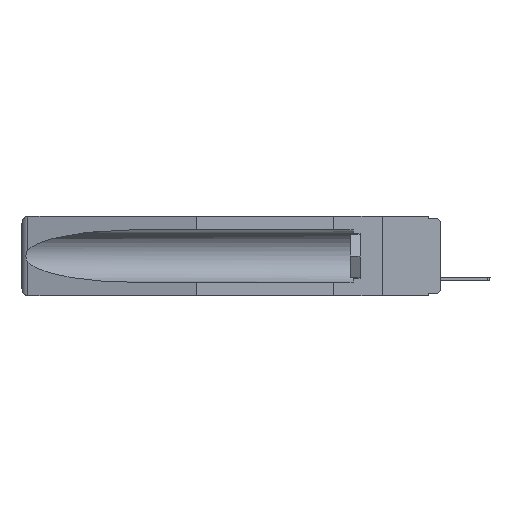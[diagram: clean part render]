
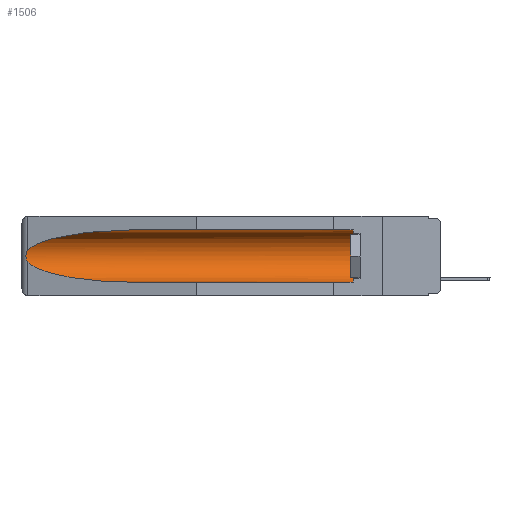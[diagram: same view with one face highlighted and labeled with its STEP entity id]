
A CAD part, left-side view. The second image highlights one B-rep face of the part: STEP entity #1506.
In plain terms, the highlighted cylindrical face has radius 2.857 mm (diameter 5.715 mm), a partial arc.
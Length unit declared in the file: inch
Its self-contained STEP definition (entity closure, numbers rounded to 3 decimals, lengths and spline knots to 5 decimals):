
#225 = EDGE_LOOP ( 'NONE', ( #8158, #10913, #3155, #18126, #15977, #18020 ) ) ;
#439 = CARTESIAN_POINT ( 'NONE',  ( 0.155, -0.30754, -0.1715 ) ) ;
#495 = VECTOR ( 'NONE', #9731, 39.37008 ) ;
#698 = VERTEX_POINT ( 'NONE', #2184 ) ;
#1495 = B_SPLINE_CURVE_WITH_KNOTS ( 'NONE', 3,
 ( #19013, #11004, #4889, #17435, #8050, #17637, #9513, #11315, #9321, #3001 ),
 .UNSPECIFIED., .F., .F.,
 ( 4, 2, 2, 2, 4 ),
 ( 0., 0.00029, 0.00058, 0.00087, 0.00117 ),
 .UNSPECIFIED. ) ;
#1506 = ADVANCED_FACE ( 'NONE', ( #10110 ), #15174, .F. ) ;
#1785 = VERTEX_POINT ( 'NONE', #9872 ) ;
#1948 =( BOUNDED_CURVE ( )  B_SPLINE_CURVE ( 3, ( #9171, #2658, #17506, #13929 ),
 .UNSPECIFIED., .F., .T. ) 
 B_SPLINE_CURVE_WITH_KNOTS ( ( 4, 4 ),
 ( 4.71239, 6.08839 ),
 .UNSPECIFIED. ) 
 CURVE ( )  GEOMETRIC_REPRESENTATION_ITEM ( )  RATIONAL_B_SPLINE_CURVE ( ( 1., 0.848, 0.848, 1. ) ) 
 REPRESENTATION_ITEM ( '' )  );
#2184 = CARTESIAN_POINT ( 'NONE',  ( 0.26537, 1.52718, -0.19328 ) ) ;
#2658 = CARTESIAN_POINT ( 'NONE',  ( 0.21114, 1.30732, -0.059 ) ) ;
#3001 = CARTESIAN_POINT ( 'NONE',  ( 0.26537, 1.52718, -0.19328 ) ) ;
#3155 = ORIENTED_EDGE ( 'NONE', *, *, #18016, .T. ) ;
#3371 = EDGE_CURVE ( 'NONE', #20706, #1785, #8905, .T. ) ;
#3880 = CARTESIAN_POINT ( 'NONE',  ( 0.25451, 1.48313, -0.24835 ) ) ;
#4019 = DIRECTION ( 'NONE',  ( 0., 1., 0. ) ) ;
#4889 = CARTESIAN_POINT ( 'NONE',  ( 0.26654, 1.53092, -0.15636 ) ) ;
#5355 = EDGE_CURVE ( 'NONE', #11355, #698, #1495, .T. ) ;
#6370 = CARTESIAN_POINT ( 'NONE',  ( 0.155, 1.07973, -0.284 ) ) ;
#6860 = DIRECTION ( 'NONE',  ( 0., 0., 1. ) ) ;
#7137 = CARTESIAN_POINT ( 'NONE',  ( 0.21114, 1.30732, -0.284 ) ) ;
#7166 = AXIS2_PLACEMENT_3D ( 'NONE', #439, #4019, #6860 ) ;
#7310 = EDGE_CURVE ( 'NONE', #20706, #19243, #8266, .T. ) ;
#7589 = EDGE_CURVE ( 'NONE', #16538, #11355, #1948, .T. ) ;
#7983 = CARTESIAN_POINT ( 'NONE',  ( 0.155, 1.07973, -0.059 ) ) ;
#8035 = LINE ( 'NONE', #16051, #13643 ) ;
#8050 = CARTESIAN_POINT ( 'NONE',  ( 0.2675, 1.53308, -0.16763 ) ) ;
#8158 = ORIENTED_EDGE ( 'NONE', *, *, #7589, .T. ) ;
#8266 = LINE ( 'NONE', #17845, #495 ) ;
#8820 = CARTESIAN_POINT ( 'NONE',  ( 0.26537, 1.52718, -0.19328 ) ) ;
#8905 = CIRCLE ( 'NONE', #10238, 0.1125 ) ;
#9171 = CARTESIAN_POINT ( 'NONE',  ( 0.155, 1.07973, -0.059 ) ) ;
#9321 = CARTESIAN_POINT ( 'NONE',  ( 0.26597, 1.5296, -0.19026 ) ) ;
#9513 = CARTESIAN_POINT ( 'NONE',  ( 0.2673, 1.53269, -0.17917 ) ) ;
#9731 = DIRECTION ( 'NONE',  ( 0., 1., 0. ) ) ;
#9872 = CARTESIAN_POINT ( 'NONE',  ( 0.155, 0.126, -0.059 ) ) ;
#10110 = FACE_OUTER_BOUND ( 'NONE', #225, .T. ) ;
#10238 = AXIS2_PLACEMENT_3D ( 'NONE', #18301, #14626, #19668 ) ;
#10538 =( BOUNDED_CURVE ( )  B_SPLINE_CURVE ( 3, ( #8820, #3880, #7137, #15049 ),
 .UNSPECIFIED., .F., .T. ) 
 B_SPLINE_CURVE_WITH_KNOTS ( ( 4, 4 ),
 ( 0.1948, 1.5708 ),
 .UNSPECIFIED. ) 
 CURVE ( )  GEOMETRIC_REPRESENTATION_ITEM ( )  RATIONAL_B_SPLINE_CURVE ( ( 1., 0.848, 0.848, 1. ) ) 
 REPRESENTATION_ITEM ( '' )  );
#10913 = ORIENTED_EDGE ( 'NONE', *, *, #5355, .T. ) ;
#11004 = CARTESIAN_POINT ( 'NONE',  ( 0.26597, 1.52961, -0.15275 ) ) ;
#11315 = CARTESIAN_POINT ( 'NONE',  ( 0.26655, 1.53094, -0.18657 ) ) ;
#11355 = VERTEX_POINT ( 'NONE', #18070 ) ;
#11617 = EDGE_CURVE ( 'NONE', #1785, #16538, #8035, .T. ) ;
#12993 = DIRECTION ( 'NONE',  ( 0., 1., 0. ) ) ;
#13643 = VECTOR ( 'NONE', #12993, 39.37008 ) ;
#13929 = CARTESIAN_POINT ( 'NONE',  ( 0.26537, 1.52718, -0.14972 ) ) ;
#14626 = DIRECTION ( 'NONE',  ( 0., -1., 0. ) ) ;
#15049 = CARTESIAN_POINT ( 'NONE',  ( 0.155, 1.07973, -0.284 ) ) ;
#15174 = CYLINDRICAL_SURFACE ( 'NONE', #7166, 0.1125 ) ;
#15977 = ORIENTED_EDGE ( 'NONE', *, *, #3371, .T. ) ;
#16051 = CARTESIAN_POINT ( 'NONE',  ( 0.155, -0.30754, -0.059 ) ) ;
#16538 = VERTEX_POINT ( 'NONE', #7983 ) ;
#16702 = CARTESIAN_POINT ( 'NONE',  ( 0.155, 0.126, -0.284 ) ) ;
#17435 = CARTESIAN_POINT ( 'NONE',  ( 0.2673, 1.5327, -0.16383 ) ) ;
#17506 = CARTESIAN_POINT ( 'NONE',  ( 0.25451, 1.48313, -0.09465 ) ) ;
#17637 = CARTESIAN_POINT ( 'NONE',  ( 0.2675, 1.53308, -0.17534 ) ) ;
#17845 = CARTESIAN_POINT ( 'NONE',  ( 0.155, -0.30754, -0.284 ) ) ;
#18016 = EDGE_CURVE ( 'NONE', #698, #19243, #10538, .T. ) ;
#18020 = ORIENTED_EDGE ( 'NONE', *, *, #11617, .T. ) ;
#18070 = CARTESIAN_POINT ( 'NONE',  ( 0.26537, 1.52718, -0.14972 ) ) ;
#18126 = ORIENTED_EDGE ( 'NONE', *, *, #7310, .F. ) ;
#18301 = CARTESIAN_POINT ( 'NONE',  ( 0.155, 0.126, -0.1715 ) ) ;
#19013 = CARTESIAN_POINT ( 'NONE',  ( 0.26537, 1.52718, -0.14972 ) ) ;
#19243 = VERTEX_POINT ( 'NONE', #6370 ) ;
#19668 = DIRECTION ( 'NONE',  ( 0., 0., 1. ) ) ;
#20706 = VERTEX_POINT ( 'NONE', #16702 ) ;
